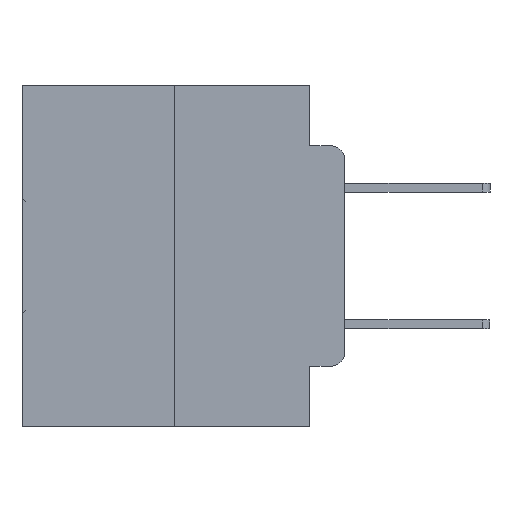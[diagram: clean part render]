
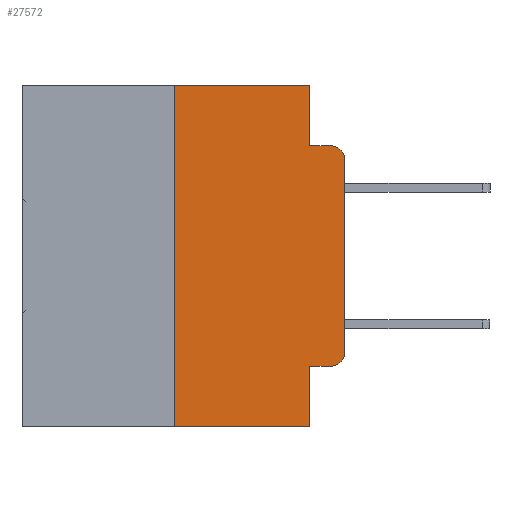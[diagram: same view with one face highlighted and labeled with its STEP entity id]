
A CAD part, left-side view. The second image highlights one B-rep face of the part: STEP entity #27572.
In plain terms, the highlighted planar face has unit normal (-1, 0, 0).
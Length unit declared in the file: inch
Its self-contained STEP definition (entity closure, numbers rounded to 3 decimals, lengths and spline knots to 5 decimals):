
#75 = ORIENTED_EDGE ( 'NONE', *, *, #17927, .T. ) ;
#635 = CARTESIAN_POINT ( 'NONE',  ( 0., 0.473, -0.5 ) ) ;
#713 = VECTOR ( 'NONE', #21721, 39.37008 ) ;
#929 = CARTESIAN_POINT ( 'NONE',  ( 0., 0.02, -0.3915 ) ) ;
#1447 = CARTESIAN_POINT ( 'NONE',  ( 0., 0.25, 0. ) ) ;
#1832 = CARTESIAN_POINT ( 'NONE',  ( 0., 0.473, 0. ) ) ;
#2711 = CARTESIAN_POINT ( 'NONE',  ( 0., 0.051, -0.4115 ) ) ;
#3376 = DIRECTION ( 'NONE',  ( 0., 0., -1. ) ) ;
#3701 = ORIENTED_EDGE ( 'NONE', *, *, #25427, .F. ) ;
#3958 = LINE ( 'NONE', #12511, #25134 ) ;
#4355 = DIRECTION ( 'NONE',  ( 0., -1., 0. ) ) ;
#4716 = CARTESIAN_POINT ( 'NONE',  ( 0., 0.02, -0.4115 ) ) ;
#5190 = FACE_OUTER_BOUND ( 'NONE', #29227, .T. ) ;
#5670 = CARTESIAN_POINT ( 'NONE',  ( 0., 0.25, 0. ) ) ;
#5749 = CIRCLE ( 'NONE', #22502, 0.02 ) ;
#5837 = EDGE_CURVE ( 'NONE', #15419, #30222, #15869, .T. ) ;
#6539 = CARTESIAN_POINT ( 'NONE',  ( 0., 0.051, 0. ) ) ;
#6569 = EDGE_CURVE ( 'NONE', #15419, #29960, #9218, .T. ) ;
#7226 = VECTOR ( 'NONE', #4355, 39.37008 ) ;
#7375 = CARTESIAN_POINT ( 'NONE',  ( 0., 0., -0.1085 ) ) ;
#7650 = DIRECTION ( 'NONE',  ( 0., -1., 0. ) ) ;
#7907 = CARTESIAN_POINT ( 'NONE',  ( 0., 0.473, 0. ) ) ;
#8050 = DIRECTION ( 'NONE',  ( 0., -1., 0. ) ) ;
#8094 = DIRECTION ( 'NONE',  ( -1., 0., 0. ) ) ;
#8126 = DIRECTION ( 'NONE',  ( 0., 0., 1. ) ) ;
#8567 = LINE ( 'NONE', #6539, #20365 ) ;
#9113 = AXIS2_PLACEMENT_3D ( 'NONE', #929, #17702, #3376 ) ;
#9218 = LINE ( 'NONE', #2711, #16200 ) ;
#11351 = VERTEX_POINT ( 'NONE', #7375 ) ;
#12129 = CARTESIAN_POINT ( 'NONE',  ( 0., 0.051, 0. ) ) ;
#12511 = CARTESIAN_POINT ( 'NONE',  ( 0., 0., 0. ) ) ;
#12638 = DIRECTION ( 'NONE',  ( 0., 0., -1. ) ) ;
#12922 = EDGE_CURVE ( 'NONE', #29960, #20271, #13676, .T. ) ;
#13271 = ORIENTED_EDGE ( 'NONE', *, *, #22313, .T. ) ;
#13503 = LINE ( 'NONE', #1832, #7226 ) ;
#13676 = CIRCLE ( 'NONE', #9113, 0.02 ) ;
#13802 = VECTOR ( 'NONE', #8050, 39.37008 ) ;
#14564 = CARTESIAN_POINT ( 'NONE',  ( 0., 0.051, -0.0885 ) ) ;
#14719 = VERTEX_POINT ( 'NONE', #22815 ) ;
#14826 = ORIENTED_EDGE ( 'NONE', *, *, #5837, .F. ) ;
#15121 = CARTESIAN_POINT ( 'NONE',  ( 0., 0.051, -0.5 ) ) ;
#15419 = VERTEX_POINT ( 'NONE', #18225 ) ;
#15528 = EDGE_CURVE ( 'NONE', #20729, #24459, #13503, .T. ) ;
#15611 = VERTEX_POINT ( 'NONE', #18830 ) ;
#15869 = LINE ( 'NONE', #12129, #22910 ) ;
#15896 = ORIENTED_EDGE ( 'NONE', *, *, #19153, .T. ) ;
#16037 = VERTEX_POINT ( 'NONE', #22847 ) ;
#16200 = VECTOR ( 'NONE', #7650, 39.37008 ) ;
#17702 = DIRECTION ( 'NONE',  ( -1., 0., 0. ) ) ;
#17927 = EDGE_CURVE ( 'NONE', #16037, #30222, #26327, .T. ) ;
#18032 = CARTESIAN_POINT ( 'NONE',  ( 0., 0.051, 0. ) ) ;
#18225 = CARTESIAN_POINT ( 'NONE',  ( 0., 0.051, -0.4115 ) ) ;
#18395 = ORIENTED_EDGE ( 'NONE', *, *, #30221, .F. ) ;
#18830 = CARTESIAN_POINT ( 'NONE',  ( 0., 0.02, -0.0885 ) ) ;
#19153 = EDGE_CURVE ( 'NONE', #20271, #11351, #3958, .T. ) ;
#20271 = VERTEX_POINT ( 'NONE', #28138 ) ;
#20365 = VECTOR ( 'NONE', #27751, 39.37008 ) ;
#20703 = ORIENTED_EDGE ( 'NONE', *, *, #15528, .F. ) ;
#20729 = VERTEX_POINT ( 'NONE', #1447 ) ;
#21721 = DIRECTION ( 'NONE',  ( 0., -1., 0. ) ) ;
#21825 = CARTESIAN_POINT ( 'NONE',  ( 0., 0.02, -0.1085 ) ) ;
#22313 = EDGE_CURVE ( 'NONE', #11351, #15611, #5749, .T. ) ;
#22502 = AXIS2_PLACEMENT_3D ( 'NONE', #21825, #8094, #24552 ) ;
#22815 = CARTESIAN_POINT ( 'NONE',  ( 0., 0.051, -0.0885 ) ) ;
#22847 = CARTESIAN_POINT ( 'NONE',  ( 0., 0.25, -0.5 ) ) ;
#22910 = VECTOR ( 'NONE', #26220, 39.37008 ) ;
#23954 = PLANE ( 'NONE',  #24368 ) ;
#24368 = AXIS2_PLACEMENT_3D ( 'NONE', #7907, #26733, #12638 ) ;
#24459 = VERTEX_POINT ( 'NONE', #18032 ) ;
#24552 = DIRECTION ( 'NONE',  ( 0., 0., -1. ) ) ;
#25134 = VECTOR ( 'NONE', #26606, 39.37008 ) ;
#25427 = EDGE_CURVE ( 'NONE', #14719, #15611, #26053, .T. ) ;
#26053 = LINE ( 'NONE', #14564, #713 ) ;
#26220 = DIRECTION ( 'NONE',  ( 0., 0., -1. ) ) ;
#26327 = LINE ( 'NONE', #635, #13802 ) ;
#26606 = DIRECTION ( 'NONE',  ( 0., 0., 1. ) ) ;
#26733 = DIRECTION ( 'NONE',  ( 1., 0., 0. ) ) ;
#27572 = ADVANCED_FACE ( 'NONE', ( #5190 ), #23954, .F. ) ;
#27623 = ORIENTED_EDGE ( 'NONE', *, *, #6569, .T. ) ;
#27751 = DIRECTION ( 'NONE',  ( 0., 0., -1. ) ) ;
#28134 = VECTOR ( 'NONE', #8126, 39.37008 ) ;
#28138 = CARTESIAN_POINT ( 'NONE',  ( 0., 0., -0.3915 ) ) ;
#28555 = EDGE_CURVE ( 'NONE', #24459, #14719, #8567, .T. ) ;
#28859 = LINE ( 'NONE', #5670, #28134 ) ;
#29227 = EDGE_LOOP ( 'NONE', ( #15896, #13271, #3701, #29461, #20703, #18395, #75, #14826, #27623, #29876 ) ) ;
#29461 = ORIENTED_EDGE ( 'NONE', *, *, #28555, .F. ) ;
#29876 = ORIENTED_EDGE ( 'NONE', *, *, #12922, .T. ) ;
#29960 = VERTEX_POINT ( 'NONE', #4716 ) ;
#30221 = EDGE_CURVE ( 'NONE', #16037, #20729, #28859, .T. ) ;
#30222 = VERTEX_POINT ( 'NONE', #15121 ) ;
